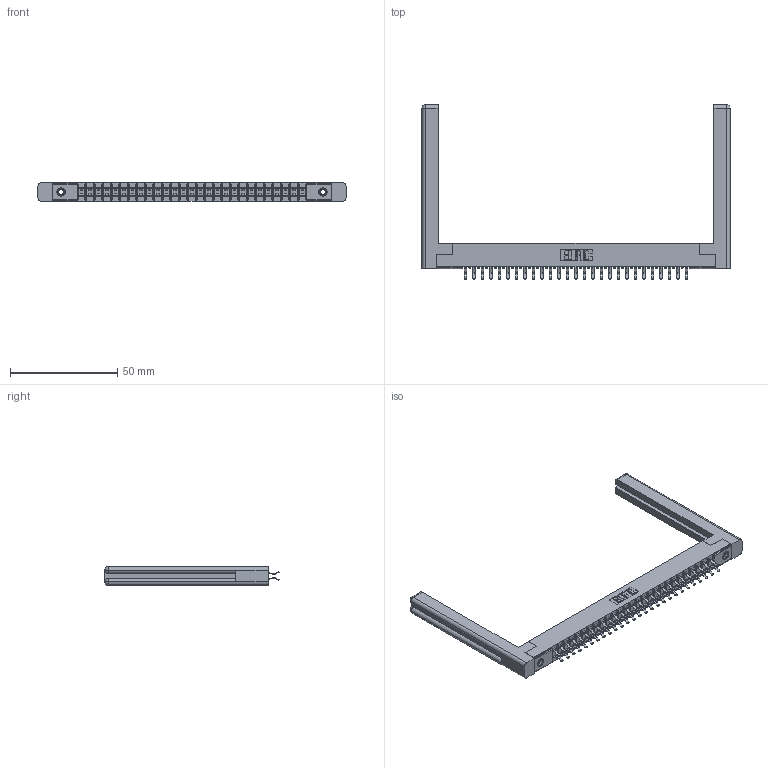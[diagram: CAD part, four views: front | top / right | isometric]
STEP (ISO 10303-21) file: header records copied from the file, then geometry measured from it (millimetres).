
FILE_DESCRIPTION (( 'STEP AP203' ), '1' );
FILE_NAME ('355-054-556-558.STEP', '2019-09-11T17:24:19', ( '' ), ( '' ), 'SwSTEP 2.0', 'SolidWorks 2016', '' );
FILE_SCHEMA (( 'CONFIG_CONTROL_DESIGN' ));
Length unit declared in the file: inch
Products named in the file (5): 307-220-058; 355-054-556-558; 345-250-001_345-250-001-102; 305 Part_.156 Dia; 305-290-001_556
Assembly tree (59 placements, depth 2):
  355-054-556-558
    305 Part_.156 Dia
    305-290-001_556  x54
    345-250-001_345-250-001-102  x2
    307-220-058  x2
Bounding box: 143.61 x 81.28 x 8.71 mm (x, y, z)
Volume: 16339.3 mm3; surface area: 22468.7 mm2
Topology: 59 solids, 59 shells, 3282 faces, 9391 edges, 6102 vertices
Faces by surface type: plane 1826, cylinder 1324, sphere 108, cone 12, torus 12
Entity records: 33915 total; most frequent: CARTESIAN_POINT 5630, ORIENTED_EDGE 5528, DIRECTION 5424, EDGE_CURVE 2764, LINE 2204, VECTOR 2204, VERTEX_POINT 1762, AXIS2_PLACEMENT_3D 1610
